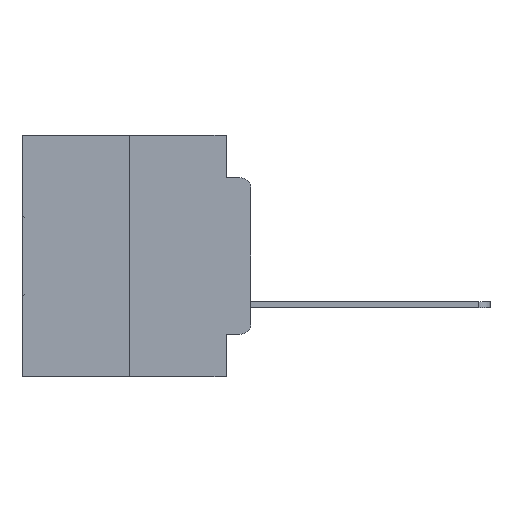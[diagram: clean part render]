
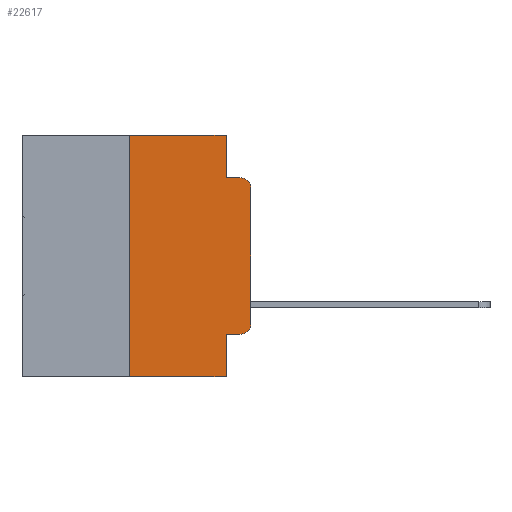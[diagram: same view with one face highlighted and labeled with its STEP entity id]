
A CAD part, left-side view. The second image highlights one B-rep face of the part: STEP entity #22617.
In plain terms, the highlighted planar face has unit normal (-1, 0, 0).
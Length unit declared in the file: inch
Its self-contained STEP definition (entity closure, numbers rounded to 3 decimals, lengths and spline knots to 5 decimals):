
#679 = EDGE_CURVE ( 'NONE', #19798, #13846, #15197, .T. ) ;
#1801 = VERTEX_POINT ( 'NONE', #24721 ) ;
#2102 = LINE ( 'NONE', #23662, #14655 ) ;
#2341 = VERTEX_POINT ( 'NONE', #26740 ) ;
#2756 = CARTESIAN_POINT ( 'NONE',  ( 0., 0.051, -0.4115 ) ) ;
#3306 = CARTESIAN_POINT ( 'NONE',  ( 0., 0.051, 0. ) ) ;
#4683 = CARTESIAN_POINT ( 'NONE',  ( 0., 0.02, -0.1085 ) ) ;
#4842 = LINE ( 'NONE', #9597, #23667 ) ;
#5219 = EDGE_CURVE ( 'NONE', #7386, #19798, #18684, .T. ) ;
#5272 = EDGE_CURVE ( 'NONE', #6599, #18558, #29187, .T. ) ;
#6599 = VERTEX_POINT ( 'NONE', #16339 ) ;
#7031 = EDGE_CURVE ( 'NONE', #13290, #10631, #4842, .T. ) ;
#7169 = ORIENTED_EDGE ( 'NONE', *, *, #5219, .T. ) ;
#7228 = DIRECTION ( 'NONE',  ( 0., 0., -1. ) ) ;
#7386 = VERTEX_POINT ( 'NONE', #15776 ) ;
#7756 = VECTOR ( 'NONE', #20076, 39.37008 ) ;
#8201 = VECTOR ( 'NONE', #23038, 39.37008 ) ;
#9035 = ORIENTED_EDGE ( 'NONE', *, *, #679, .T. ) ;
#9349 = CARTESIAN_POINT ( 'NONE',  ( 0., 0.25, -0.5 ) ) ;
#9440 = EDGE_CURVE ( 'NONE', #1801, #10631, #30435, .T. ) ;
#9597 = CARTESIAN_POINT ( 'NONE',  ( 0., 0.473, -0.5 ) ) ;
#9937 = VECTOR ( 'NONE', #30453, 39.37008 ) ;
#10197 = PLANE ( 'NONE',  #11952 ) ;
#10631 = VERTEX_POINT ( 'NONE', #13716 ) ;
#11952 = AXIS2_PLACEMENT_3D ( 'NONE', #19780, #29497, #15103 ) ;
#12778 = CARTESIAN_POINT ( 'NONE',  ( 0., 0.051, 0. ) ) ;
#13290 = VERTEX_POINT ( 'NONE', #9349 ) ;
#13564 = CARTESIAN_POINT ( 'NONE',  ( 0., 0.02, -0.3915 ) ) ;
#13716 = CARTESIAN_POINT ( 'NONE',  ( 0., 0.051, -0.5 ) ) ;
#13846 = VERTEX_POINT ( 'NONE', #28346 ) ;
#13978 = LINE ( 'NONE', #3306, #8201 ) ;
#13995 = EDGE_CURVE ( 'NONE', #13846, #18558, #26565, .T. ) ;
#14116 = ORIENTED_EDGE ( 'NONE', *, *, #23539, .F. ) ;
#14435 = LINE ( 'NONE', #18749, #19347 ) ;
#14655 = VECTOR ( 'NONE', #26034, 39.37008 ) ;
#15103 = DIRECTION ( 'NONE',  ( 0., 0., -1. ) ) ;
#15110 = DIRECTION ( 'NONE',  ( 0., 0., 1. ) ) ;
#15197 = LINE ( 'NONE', #31897, #20123 ) ;
#15642 = ORIENTED_EDGE ( 'NONE', *, *, #7031, .T. ) ;
#15776 = CARTESIAN_POINT ( 'NONE',  ( 0., 0.02, -0.4115 ) ) ;
#15977 = DIRECTION ( 'NONE',  ( 0., 0., -1. ) ) ;
#16339 = CARTESIAN_POINT ( 'NONE',  ( 0., 0.051, -0.0885 ) ) ;
#16384 = VERTEX_POINT ( 'NONE', #29009 ) ;
#17198 = FACE_OUTER_BOUND ( 'NONE', #19790, .T. ) ;
#18558 = VERTEX_POINT ( 'NONE', #19920 ) ;
#18684 = CIRCLE ( 'NONE', #23400, 0.02 ) ;
#18749 = CARTESIAN_POINT ( 'NONE',  ( 0., 0.25, 0. ) ) ;
#19347 = VECTOR ( 'NONE', #28395, 39.37008 ) ;
#19674 = EDGE_CURVE ( 'NONE', #16384, #6599, #13978, .T. ) ;
#19780 = CARTESIAN_POINT ( 'NONE',  ( 0., 0.473, 0. ) ) ;
#19790 = EDGE_LOOP ( 'NONE', ( #9035, #23551, #23235, #23984, #25479, #14116, #15642, #23622, #31406, #7169 ) ) ;
#19798 = VERTEX_POINT ( 'NONE', #30008 ) ;
#19920 = CARTESIAN_POINT ( 'NONE',  ( 0., 0.02, -0.0885 ) ) ;
#20076 = DIRECTION ( 'NONE',  ( 0., -1., 0. ) ) ;
#20123 = VECTOR ( 'NONE', #15110, 39.37008 ) ;
#20606 = EDGE_CURVE ( 'NONE', #2341, #16384, #2102, .T. ) ;
#20765 = LINE ( 'NONE', #2756, #7756 ) ;
#21890 = DIRECTION ( 'NONE',  ( -1., 0., 0. ) ) ;
#22617 = ADVANCED_FACE ( 'NONE', ( #17198 ), #10197, .F. ) ;
#23038 = DIRECTION ( 'NONE',  ( 0., 0., -1. ) ) ;
#23235 = ORIENTED_EDGE ( 'NONE', *, *, #5272, .F. ) ;
#23400 = AXIS2_PLACEMENT_3D ( 'NONE', #13564, #30362, #15977 ) ;
#23539 = EDGE_CURVE ( 'NONE', #13290, #2341, #14435, .T. ) ;
#23551 = ORIENTED_EDGE ( 'NONE', *, *, #13995, .T. ) ;
#23622 = ORIENTED_EDGE ( 'NONE', *, *, #9440, .F. ) ;
#23662 = CARTESIAN_POINT ( 'NONE',  ( 0., 0.473, 0. ) ) ;
#23667 = VECTOR ( 'NONE', #24178, 39.37008 ) ;
#23984 = ORIENTED_EDGE ( 'NONE', *, *, #19674, .F. ) ;
#24178 = DIRECTION ( 'NONE',  ( 0., -1., 0. ) ) ;
#24721 = CARTESIAN_POINT ( 'NONE',  ( 0., 0.051, -0.4115 ) ) ;
#25319 = EDGE_CURVE ( 'NONE', #1801, #7386, #20765, .T. ) ;
#25479 = ORIENTED_EDGE ( 'NONE', *, *, #20606, .F. ) ;
#26034 = DIRECTION ( 'NONE',  ( 0., -1., 0. ) ) ;
#26530 = AXIS2_PLACEMENT_3D ( 'NONE', #4683, #21890, #7228 ) ;
#26565 = CIRCLE ( 'NONE', #26530, 0.02 ) ;
#26740 = CARTESIAN_POINT ( 'NONE',  ( 0., 0.25, 0. ) ) ;
#27228 = DIRECTION ( 'NONE',  ( 0., 0., -1. ) ) ;
#28077 = CARTESIAN_POINT ( 'NONE',  ( 0., 0.051, -0.0885 ) ) ;
#28346 = CARTESIAN_POINT ( 'NONE',  ( 0., 0., -0.1085 ) ) ;
#28395 = DIRECTION ( 'NONE',  ( 0., 0., 1. ) ) ;
#29009 = CARTESIAN_POINT ( 'NONE',  ( 0., 0.051, 0. ) ) ;
#29187 = LINE ( 'NONE', #28077, #9937 ) ;
#29497 = DIRECTION ( 'NONE',  ( 1., 0., 0. ) ) ;
#29709 = VECTOR ( 'NONE', #27228, 39.37008 ) ;
#30008 = CARTESIAN_POINT ( 'NONE',  ( 0., 0., -0.3915 ) ) ;
#30362 = DIRECTION ( 'NONE',  ( -1., 0., 0. ) ) ;
#30435 = LINE ( 'NONE', #12778, #29709 ) ;
#30453 = DIRECTION ( 'NONE',  ( 0., -1., 0. ) ) ;
#31406 = ORIENTED_EDGE ( 'NONE', *, *, #25319, .T. ) ;
#31897 = CARTESIAN_POINT ( 'NONE',  ( 0., 0., 0. ) ) ;
